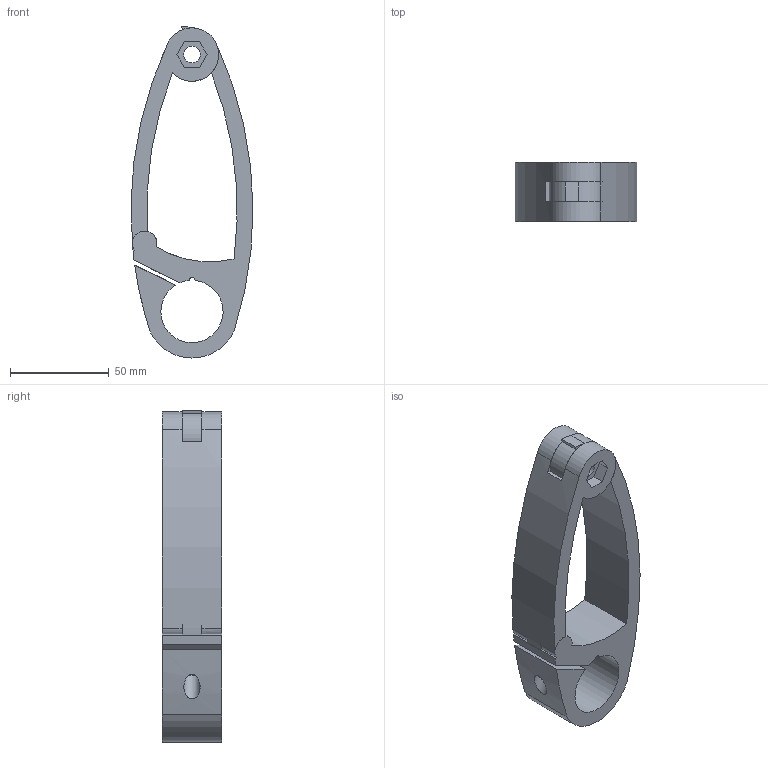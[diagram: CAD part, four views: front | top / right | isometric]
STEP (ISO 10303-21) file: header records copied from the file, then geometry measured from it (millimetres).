
FILE_DESCRIPTION(/* description */ (''),/* implementation_level */ '2;1');
FILE_NAME(/* name */ 'Tailhook-Mod-1-1 v1.step',/* time_stamp */ '2018-00-00T00:00:00-00:00',/* author */ ('fosscadbot'),/* organization */ (''),/* preprocessor_version */ 'ST-DEVELOPER v17',/* originating_system */ 'Autodesk Translation Framework v7.1.0.215',/* authorisation */ '');
FILE_SCHEMA (('AUTOMOTIVE_DESIGN { 1 0 10303 214 3 1 1 }'));
Length unit declared in the file: millimetre
Products named in the file (3): Tailhook-Mod-1; Component1; Component2
Assembly tree (2 placements, depth 2):
  Tailhook-Mod-1
    Component1
    Component2
Bounding box: 61.7 x 30 x 167.95 mm (x, y, z)
Volume: 109052.5 mm3; surface area: 36086.4 mm2
Topology: 2 solids, 2 shells, 63 faces, 158 edges, 101 vertices
Faces by surface type: cylinder 32, plane 31
Full cylindrical faces by diameter (mm): 3 x2, 8.2 x1, 8.5 x3
Entity records: 2084 total; most frequent: CARTESIAN_POINT 403, DIRECTION 360, ORIENTED_EDGE 318, EDGE_CURVE 159, AXIS2_PLACEMENT_3D 136, VERTEX_POINT 101, LINE 88, VECTOR 88
